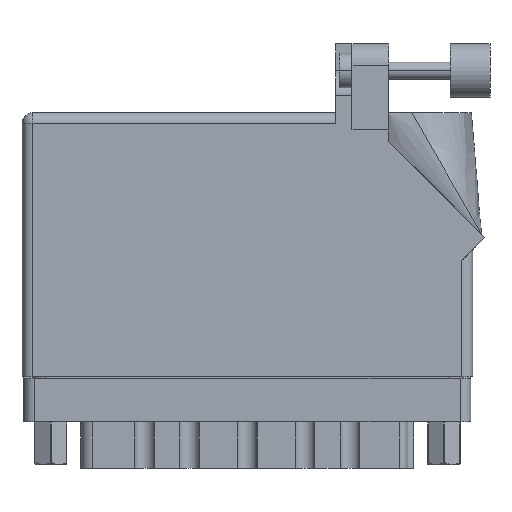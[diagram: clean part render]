
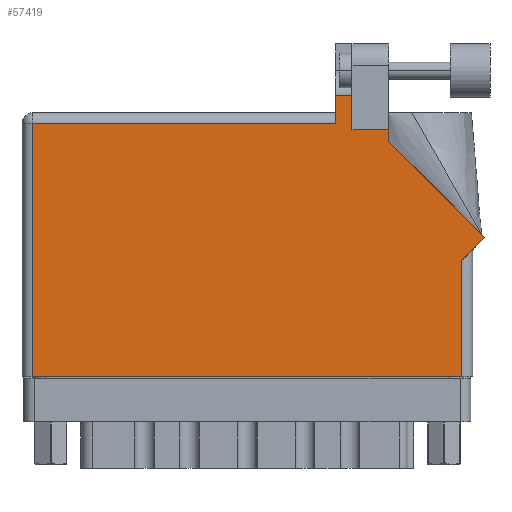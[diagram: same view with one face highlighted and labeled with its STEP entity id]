
A CAD part, front view. The second image highlights one B-rep face of the part: STEP entity #57419.
In plain terms, the highlighted face is planar.
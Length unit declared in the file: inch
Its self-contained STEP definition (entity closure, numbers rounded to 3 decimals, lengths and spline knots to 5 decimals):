
#1293 = CARTESIAN_POINT ( 'NONE',  ( 2.126, 1.36442, 0. ) ) ;
#1773 = CARTESIAN_POINT ( 'NONE',  ( 2.24377, 1.6315, 0. ) ) ;
#2945 = VECTOR ( 'NONE', #10519, 39.37008 ) ;
#2980 = DIRECTION ( 'NONE',  ( 1., 0., 0. ) ) ;
#7391 = LINE ( 'NONE', #52805, #57242 ) ;
#7632 = CARTESIAN_POINT ( 'NONE',  ( 2.55, 0.675, 0. ) ) ;
#8299 = VECTOR ( 'NONE', #49128, 39.37008 ) ;
#8927 = DIRECTION ( 'NONE',  ( 0., -1., 0. ) ) ;
#10492 = ORIENTED_EDGE ( 'NONE', *, *, #23031, .T. ) ;
#10500 = CARTESIAN_POINT ( 'NONE',  ( 1.819, 1.468, 0. ) ) ;
#10519 = DIRECTION ( 'NONE',  ( 0., 1., 0. ) ) ;
#12210 = LINE ( 'NONE', #39096, #21230 ) ;
#12682 = VERTEX_POINT ( 'NONE', #45704 ) ;
#13855 = VECTOR ( 'NONE', #59432, 39.37008 ) ;
#15295 = CARTESIAN_POINT ( 'NONE',  ( 1.913, 1.6315, 0. ) ) ;
#15626 = ORIENTED_EDGE ( 'NONE', *, *, #35380, .T. ) ;
#16230 = CARTESIAN_POINT ( 'NONE',  ( 2.126, 1.36442, 0. ) ) ;
#16235 = LINE ( 'NONE', #47080, #59285 ) ;
#17546 = ORIENTED_EDGE ( 'NONE', *, *, #32854, .T. ) ;
#17811 = VERTEX_POINT ( 'NONE', #59900 ) ;
#19119 = CARTESIAN_POINT ( 'NONE',  ( 0., 1.468, 0. ) ) ;
#19362 = LINE ( 'NONE', #19119, #53326 ) ;
#19371 = EDGE_CURVE ( 'NONE', #37977, #61627, #12210, .T. ) ;
#19468 = VERTEX_POINT ( 'NONE', #1293 ) ;
#19760 = ORIENTED_EDGE ( 'NONE', *, *, #39125, .T. ) ;
#20009 = CARTESIAN_POINT ( 'NONE',  ( 2.126, 1.43, 0. ) ) ;
#20920 = VECTOR ( 'NONE', #54469, 39.37008 ) ;
#21230 = VECTOR ( 'NONE', #48806, 39.37008 ) ;
#21698 = DIRECTION ( 'NONE',  ( -0.707, 0.707, 0. ) ) ;
#23031 = EDGE_CURVE ( 'NONE', #12682, #29516, #30769, .T. ) ;
#23278 = EDGE_LOOP ( 'NONE', ( #19760, #17546, #58517, #44851, #34309, #15626, #10492, #47884, #56107, #52866, #47028 ) ) ;
#23499 = VECTOR ( 'NONE', #47380, 39.37008 ) ;
#25213 = CARTESIAN_POINT ( 'NONE',  ( 2.126, 1.43, 0. ) ) ;
#26323 = VERTEX_POINT ( 'NONE', #10500 ) ;
#27190 = CARTESIAN_POINT ( 'NONE',  ( 1.819, 1.6315, 0. ) ) ;
#28844 = LINE ( 'NONE', #36473, #52970 ) ;
#29516 = VERTEX_POINT ( 'NONE', #7632 ) ;
#29671 = CARTESIAN_POINT ( 'NONE',  ( 0.062, 1.468, 0. ) ) ;
#30465 = EDGE_CURVE ( 'NONE', #17811, #19468, #28844, .T. ) ;
#30607 = PLANE ( 'NONE',  #46047 ) ;
#30769 = LINE ( 'NONE', #33622, #20920 ) ;
#30822 = CARTESIAN_POINT ( 'NONE',  ( 0., 1.53, 0. ) ) ;
#31720 = LINE ( 'NONE', #20009, #8299 ) ;
#32520 = CARTESIAN_POINT ( 'NONE',  ( 0., 0., 0. ) ) ;
#32854 = EDGE_CURVE ( 'NONE', #45072, #40310, #45497, .T. ) ;
#33083 = LINE ( 'NONE', #32520, #44413 ) ;
#33622 = CARTESIAN_POINT ( 'NONE',  ( 2.55, 0.737, 0. ) ) ;
#34309 = ORIENTED_EDGE ( 'NONE', *, *, #19371, .T. ) ;
#35258 = DIRECTION ( 'NONE',  ( 0., 0., -1. ) ) ;
#35380 = EDGE_CURVE ( 'NONE', #61627, #12682, #33083, .T. ) ;
#35668 = DIRECTION ( 'NONE',  ( -1., 0., 0. ) ) ;
#36313 = LINE ( 'NONE', #62416, #23499 ) ;
#36466 = EDGE_CURVE ( 'NONE', #19468, #44495, #47482, .T. ) ;
#36473 = CARTESIAN_POINT ( 'NONE',  ( 2.68271, 0.80771, 0. ) ) ;
#37977 = VERTEX_POINT ( 'NONE', #29671 ) ;
#38752 = EDGE_CURVE ( 'NONE', #26323, #37977, #19362, .T. ) ;
#39096 = CARTESIAN_POINT ( 'NONE',  ( 0.062, 0., 0. ) ) ;
#39125 = EDGE_CURVE ( 'NONE', #49193, #45072, #16235, .T. ) ;
#40310 = VERTEX_POINT ( 'NONE', #27190 ) ;
#41400 = EDGE_CURVE ( 'NONE', #29516, #17811, #36313, .T. ) ;
#41815 = CARTESIAN_POINT ( 'NONE',  ( 0.062, 0., 0. ) ) ;
#44413 = VECTOR ( 'NONE', #2980, 39.37008 ) ;
#44495 = VERTEX_POINT ( 'NONE', #25213 ) ;
#44851 = ORIENTED_EDGE ( 'NONE', *, *, #38752, .T. ) ;
#45072 = VERTEX_POINT ( 'NONE', #15295 ) ;
#45497 = LINE ( 'NONE', #1773, #13855 ) ;
#45704 = CARTESIAN_POINT ( 'NONE',  ( 2.55, 0., 0. ) ) ;
#46047 = AXIS2_PLACEMENT_3D ( 'NONE', #30822, #35258, #35668 ) ;
#47028 = ORIENTED_EDGE ( 'NONE', *, *, #48117, .T. ) ;
#47080 = CARTESIAN_POINT ( 'NONE',  ( 1.913, 1.43, 0. ) ) ;
#47380 = DIRECTION ( 'NONE',  ( 0.707, 0.707, 0. ) ) ;
#47482 = LINE ( 'NONE', #16230, #2945 ) ;
#47590 = DIRECTION ( 'NONE',  ( -1., 0., 0. ) ) ;
#47884 = ORIENTED_EDGE ( 'NONE', *, *, #41400, .T. ) ;
#48117 = EDGE_CURVE ( 'NONE', #44495, #49193, #31720, .T. ) ;
#48717 = FACE_OUTER_BOUND ( 'NONE', #23278, .T. ) ;
#48806 = DIRECTION ( 'NONE',  ( 0., -1., 0. ) ) ;
#49128 = DIRECTION ( 'NONE',  ( -1., 0., 0. ) ) ;
#49193 = VERTEX_POINT ( 'NONE', #54247 ) ;
#52805 = CARTESIAN_POINT ( 'NONE',  ( 1.819, 1.53, 0. ) ) ;
#52866 = ORIENTED_EDGE ( 'NONE', *, *, #36466, .T. ) ;
#52970 = VECTOR ( 'NONE', #21698, 39.37008 ) ;
#53326 = VECTOR ( 'NONE', #47590, 39.37008 ) ;
#54247 = CARTESIAN_POINT ( 'NONE',  ( 1.913, 1.43, 0. ) ) ;
#54469 = DIRECTION ( 'NONE',  ( 0., 1., 0. ) ) ;
#55318 = EDGE_CURVE ( 'NONE', #40310, #26323, #7391, .T. ) ;
#56107 = ORIENTED_EDGE ( 'NONE', *, *, #30465, .T. ) ;
#57242 = VECTOR ( 'NONE', #8927, 39.37008 ) ;
#57419 = ADVANCED_FACE ( 'NONE', ( #48717 ), #30607, .F. ) ;
#58517 = ORIENTED_EDGE ( 'NONE', *, *, #55318, .T. ) ;
#59285 = VECTOR ( 'NONE', #61288, 39.37008 ) ;
#59432 = DIRECTION ( 'NONE',  ( -1., 0., 0. ) ) ;
#59900 = CARTESIAN_POINT ( 'NONE',  ( 2.68271, 0.80771, 0. ) ) ;
#61288 = DIRECTION ( 'NONE',  ( 0., 1., 0. ) ) ;
#61627 = VERTEX_POINT ( 'NONE', #41815 ) ;
#62416 = CARTESIAN_POINT ( 'NONE',  ( 2.612, 0.737, 0. ) ) ;
